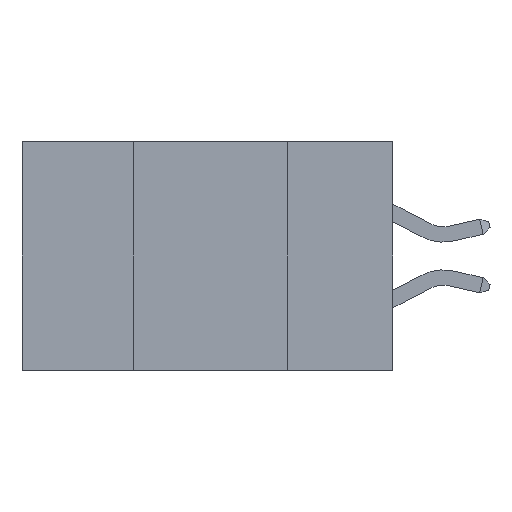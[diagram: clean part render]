
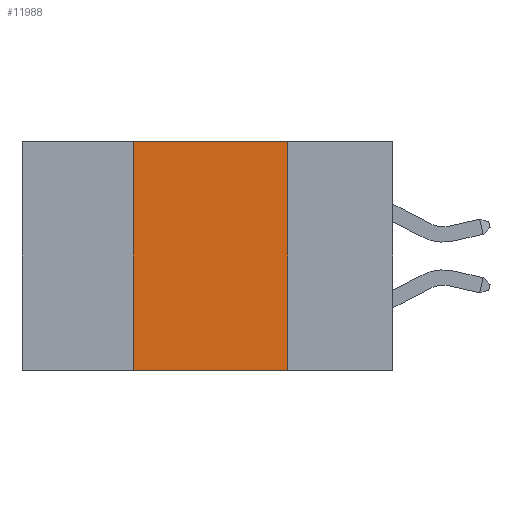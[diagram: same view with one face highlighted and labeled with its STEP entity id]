
A CAD part, left-side view. The second image highlights one B-rep face of the part: STEP entity #11988.
In plain terms, the highlighted planar face has unit normal (-1, 0, 0).
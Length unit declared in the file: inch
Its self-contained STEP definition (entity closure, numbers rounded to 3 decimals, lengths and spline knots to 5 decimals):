
#96 = VERTEX_POINT ( 'NONE', #3498 ) ;
#819 = EDGE_CURVE ( 'NONE', #11781, #3467, #16647, .T. ) ;
#829 = VERTEX_POINT ( 'NONE', #12874 ) ;
#961 = VECTOR ( 'NONE', #4338, 39.37008 ) ;
#1430 = CARTESIAN_POINT ( 'NONE',  ( 0., 0.42, -0.37 ) ) ;
#1452 = ORIENTED_EDGE ( 'NONE', *, *, #15250, .F. ) ;
#1583 = LINE ( 'NONE', #7009, #961 ) ;
#2536 = CARTESIAN_POINT ( 'NONE',  ( 0., 0.6, -0.37 ) ) ;
#3404 = PLANE ( 'NONE',  #9264 ) ;
#3467 = VERTEX_POINT ( 'NONE', #6145 ) ;
#3498 = CARTESIAN_POINT ( 'NONE',  ( 0., 0.17, -0.37 ) ) ;
#3530 = CARTESIAN_POINT ( 'NONE',  ( 0., 0.42, 0. ) ) ;
#4338 = DIRECTION ( 'NONE',  ( 0., -1., 0. ) ) ;
#4729 = FACE_OUTER_BOUND ( 'NONE', #12953, .T. ) ;
#4779 = DIRECTION ( 'NONE',  ( 1., 0., 0. ) ) ;
#6145 = CARTESIAN_POINT ( 'NONE',  ( 0., 0.42, 0. ) ) ;
#6296 = EDGE_CURVE ( 'NONE', #3467, #829, #1583, .T. ) ;
#6523 = DIRECTION ( 'NONE',  ( 0., -1., 0. ) ) ;
#7009 = CARTESIAN_POINT ( 'NONE',  ( 0., 0.6, 0. ) ) ;
#7585 = CARTESIAN_POINT ( 'NONE',  ( 0., 0.17, 0. ) ) ;
#8721 = LINE ( 'NONE', #7585, #11263 ) ;
#9044 = DIRECTION ( 'NONE',  ( 0., 0., -1. ) ) ;
#9264 = AXIS2_PLACEMENT_3D ( 'NONE', #12873, #4779, #9044 ) ;
#9689 = ORIENTED_EDGE ( 'NONE', *, *, #6296, .F. ) ;
#10310 = VECTOR ( 'NONE', #12998, 39.37008 ) ;
#11263 = VECTOR ( 'NONE', #17154, 39.37008 ) ;
#11781 = VERTEX_POINT ( 'NONE', #1430 ) ;
#11944 = LINE ( 'NONE', #2536, #15494 ) ;
#11988 = ADVANCED_FACE ( 'NONE', ( #4729 ), #3404, .F. ) ;
#12098 = ORIENTED_EDGE ( 'NONE', *, *, #12117, .T. ) ;
#12117 = EDGE_CURVE ( 'NONE', #11781, #96, #11944, .T. ) ;
#12873 = CARTESIAN_POINT ( 'NONE',  ( 0., 0.6, 0. ) ) ;
#12874 = CARTESIAN_POINT ( 'NONE',  ( 0., 0.17, 0. ) ) ;
#12953 = EDGE_LOOP ( 'NONE', ( #1452, #9689, #17337, #12098 ) ) ;
#12998 = DIRECTION ( 'NONE',  ( 0., 0., 1. ) ) ;
#15250 = EDGE_CURVE ( 'NONE', #829, #96, #8721, .T. ) ;
#15494 = VECTOR ( 'NONE', #6523, 39.37008 ) ;
#16647 = LINE ( 'NONE', #3530, #10310 ) ;
#17154 = DIRECTION ( 'NONE',  ( 0., 0., -1. ) ) ;
#17337 = ORIENTED_EDGE ( 'NONE', *, *, #819, .F. ) ;
